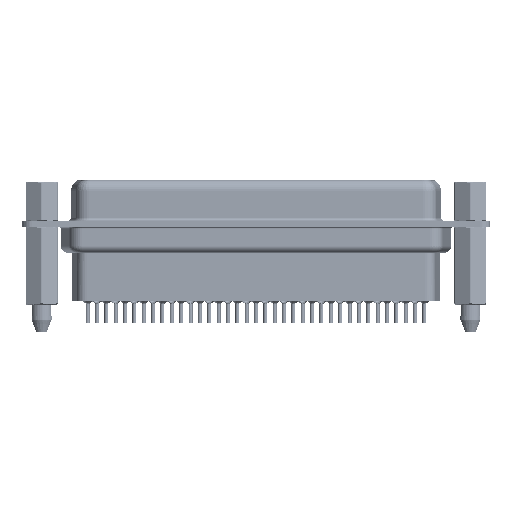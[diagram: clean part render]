
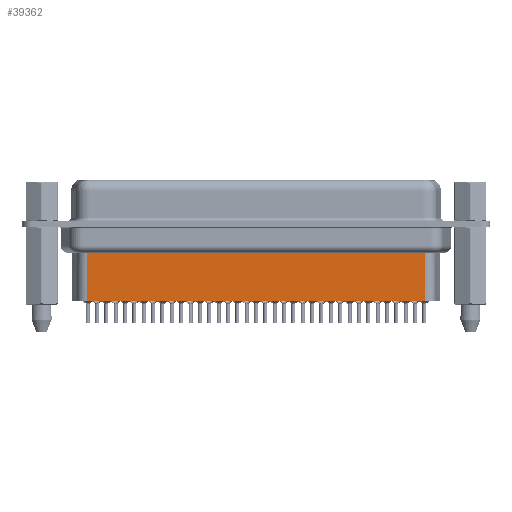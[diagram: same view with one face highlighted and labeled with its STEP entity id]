
A CAD part, front view. The second image highlights one B-rep face of the part: STEP entity #39362.
In plain terms, the highlighted planar face has unit normal (0, -1, 0).
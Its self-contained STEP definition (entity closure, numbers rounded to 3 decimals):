
#730 = CARTESIAN_POINT ( 'NONE',  ( 6.706, -3.5, -3.1 ) ) ;
#775 = CARTESIAN_POINT ( 'NONE',  ( 6.706, -3.5, -3.1 ) ) ;
#1798 = DIRECTION ( 'NONE',  ( 0., 0., -1. ) ) ;
#3502 = VECTOR ( 'NONE', #1798, 1000. ) ;
#3816 = DIRECTION ( 'NONE',  ( 1., 0., 0. ) ) ;
#5097 = EDGE_CURVE ( 'NONE', #32700, #12364, #28134, .T. ) ;
#5418 = LINE ( 'NONE', #7819, #3502 ) ;
#5973 = EDGE_CURVE ( 'NONE', #6990, #12364, #37016, .T. ) ;
#6990 = VERTEX_POINT ( 'NONE', #13887 ) ;
#7819 = CARTESIAN_POINT ( 'NONE',  ( 56.794, -3.5, -3.1 ) ) ;
#10178 = DIRECTION ( 'NONE',  ( -1., 0., 0. ) ) ;
#10200 = FACE_OUTER_BOUND ( 'NONE', #30286, .T. ) ;
#12364 = VERTEX_POINT ( 'NONE', #39163 ) ;
#12924 = VECTOR ( 'NONE', #34223, 1000. ) ;
#13887 = CARTESIAN_POINT ( 'NONE',  ( 6.706, -3.5, -4.097 ) ) ;
#16497 = LINE ( 'NONE', #34506, #36719 ) ;
#18094 = VERTEX_POINT ( 'NONE', #24793 ) ;
#19288 = ORIENTED_EDGE ( 'NONE', *, *, #5973, .T. ) ;
#20006 = ORIENTED_EDGE ( 'NONE', *, *, #5097, .F. ) ;
#21330 = CARTESIAN_POINT ( 'NONE',  ( 6.706, -3.5, -11.45 ) ) ;
#22210 = DIRECTION ( 'NONE',  ( 0., -1., 0. ) ) ;
#22530 = AXIS2_PLACEMENT_3D ( 'NONE', #730, #22210, #3816 ) ;
#24071 = ORIENTED_EDGE ( 'NONE', *, *, #34421, .T. ) ;
#24793 = CARTESIAN_POINT ( 'NONE',  ( 56.794, -3.5, -4.097 ) ) ;
#24819 = EDGE_CURVE ( 'NONE', #18094, #32700, #5418, .T. ) ;
#24981 = CARTESIAN_POINT ( 'NONE',  ( 56.794, -3.5, -11.45 ) ) ;
#27159 = VECTOR ( 'NONE', #30696, 1000. ) ;
#28134 = LINE ( 'NONE', #21330, #27159 ) ;
#30286 = EDGE_LOOP ( 'NONE', ( #34940, #24071, #19288, #20006 ) ) ;
#30696 = DIRECTION ( 'NONE',  ( -1., 0., 0. ) ) ;
#32700 = VERTEX_POINT ( 'NONE', #24981 ) ;
#34180 = PLANE ( 'NONE',  #22530 ) ;
#34223 = DIRECTION ( 'NONE',  ( 0., 0., -1. ) ) ;
#34421 = EDGE_CURVE ( 'NONE', #18094, #6990, #16497, .T. ) ;
#34506 = CARTESIAN_POINT ( 'NONE',  ( 6.459, -3.5, -4.097 ) ) ;
#34940 = ORIENTED_EDGE ( 'NONE', *, *, #24819, .F. ) ;
#36719 = VECTOR ( 'NONE', #10178, 1000. ) ;
#37016 = LINE ( 'NONE', #775, #12924 ) ;
#39163 = CARTESIAN_POINT ( 'NONE',  ( 6.706, -3.5, -11.45 ) ) ;
#39362 = ADVANCED_FACE ( 'NONE', ( #10200 ), #34180, .T. ) ;
